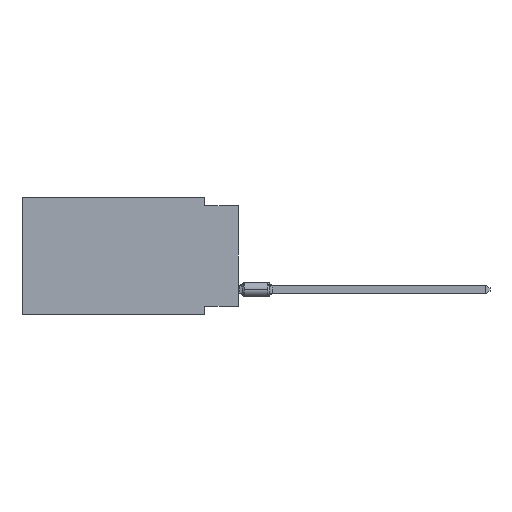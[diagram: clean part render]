
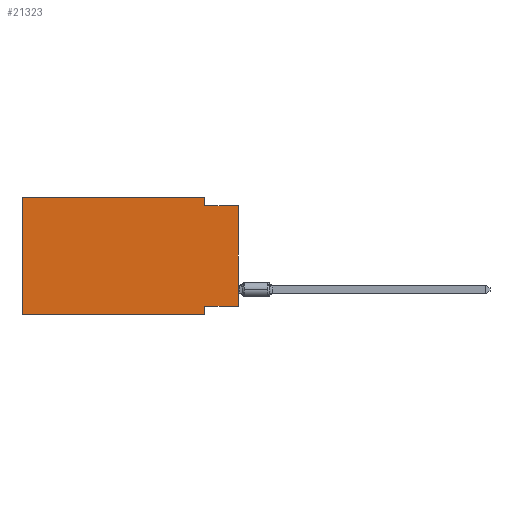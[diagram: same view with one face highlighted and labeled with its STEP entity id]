
A CAD part, left-side view. The second image highlights one B-rep face of the part: STEP entity #21323.
In plain terms, the highlighted planar face has unit normal (-1, 0, 0).
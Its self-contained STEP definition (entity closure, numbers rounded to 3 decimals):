
#197 = CARTESIAN_POINT ( 'NONE',  ( 0., 0., -0.635 ) ) ;
#879 = ORIENTED_EDGE ( 'NONE', *, *, #2220, .F. ) ;
#1951 = VECTOR ( 'NONE', #9381, 1000. ) ;
#2060 = CARTESIAN_POINT ( 'NONE',  ( 0., 2.54, -8.89 ) ) ;
#2220 = EDGE_CURVE ( 'NONE', #26242, #5443, #21758, .T. ) ;
#3222 = DIRECTION ( 'NONE',  ( 0., 0., -1. ) ) ;
#3522 = ORIENTED_EDGE ( 'NONE', *, *, #27773, .F. ) ;
#3531 = CARTESIAN_POINT ( 'NONE',  ( 0., 0., -8.255 ) ) ;
#5067 = CARTESIAN_POINT ( 'NONE',  ( 0., 16.383, 0. ) ) ;
#5443 = VERTEX_POINT ( 'NONE', #11147 ) ;
#5826 = LINE ( 'NONE', #3531, #21915 ) ;
#6061 = VERTEX_POINT ( 'NONE', #25067 ) ;
#6140 = CARTESIAN_POINT ( 'NONE',  ( 0., 0., 0. ) ) ;
#6212 = VERTEX_POINT ( 'NONE', #23338 ) ;
#6321 = VECTOR ( 'NONE', #11438, 1000. ) ;
#6931 = LINE ( 'NONE', #5067, #1951 ) ;
#7068 = CARTESIAN_POINT ( 'NONE',  ( 0., 0., -8.255 ) ) ;
#8894 = LINE ( 'NONE', #13213, #27435 ) ;
#9102 = DIRECTION ( 'NONE',  ( 0., 0., -1. ) ) ;
#9381 = DIRECTION ( 'NONE',  ( 0., 0., 1. ) ) ;
#9440 = ORIENTED_EDGE ( 'NONE', *, *, #27808, .F. ) ;
#9858 = DIRECTION ( 'NONE',  ( 0., 1., 0. ) ) ;
#10807 = VERTEX_POINT ( 'NONE', #12967 ) ;
#10947 = ORIENTED_EDGE ( 'NONE', *, *, #16075, .T. ) ;
#10988 = ORIENTED_EDGE ( 'NONE', *, *, #23152, .F. ) ;
#11147 = CARTESIAN_POINT ( 'NONE',  ( 0., 2.54, -8.89 ) ) ;
#11438 = DIRECTION ( 'NONE',  ( 0., -1., 0. ) ) ;
#12354 = VERTEX_POINT ( 'NONE', #7068 ) ;
#12698 = VECTOR ( 'NONE', #27195, 1000. ) ;
#12967 = CARTESIAN_POINT ( 'NONE',  ( 0., 16.383, 0. ) ) ;
#13213 = CARTESIAN_POINT ( 'NONE',  ( 0., 16.383, 0. ) ) ;
#13709 = EDGE_LOOP ( 'NONE', ( #16126, #23809, #3522, #10988, #9440, #10947, #879, #17304 ) ) ;
#14358 = VECTOR ( 'NONE', #27237, 1000. ) ;
#14563 = FACE_OUTER_BOUND ( 'NONE', #13709, .T. ) ;
#16075 = EDGE_CURVE ( 'NONE', #6212, #5443, #20333, .T. ) ;
#16126 = ORIENTED_EDGE ( 'NONE', *, *, #28358, .T. ) ;
#16283 = LINE ( 'NONE', #18000, #14358 ) ;
#17304 = ORIENTED_EDGE ( 'NONE', *, *, #20858, .F. ) ;
#17665 = DIRECTION ( 'NONE',  ( 0., -1., 0. ) ) ;
#17856 = VECTOR ( 'NONE', #9102, 1000. ) ;
#18000 = CARTESIAN_POINT ( 'NONE',  ( 0., 2.54, 0. ) ) ;
#18242 = AXIS2_PLACEMENT_3D ( 'NONE', #24934, #22922, #3222 ) ;
#18428 = EDGE_CURVE ( 'NONE', #20421, #21186, #18538, .T. ) ;
#18538 = LINE ( 'NONE', #20403, #12698 ) ;
#19218 = DIRECTION ( 'NONE',  ( 0., 0., 1. ) ) ;
#20333 = LINE ( 'NONE', #26401, #6321 ) ;
#20403 = CARTESIAN_POINT ( 'NONE',  ( 0., 0., -0.635 ) ) ;
#20421 = VERTEX_POINT ( 'NONE', #24693 ) ;
#20858 = EDGE_CURVE ( 'NONE', #12354, #26242, #5826, .T. ) ;
#20903 = PLANE ( 'NONE',  #18242 ) ;
#21113 = LINE ( 'NONE', #6140, #23110 ) ;
#21186 = VERTEX_POINT ( 'NONE', #197 ) ;
#21323 = ADVANCED_FACE ( 'NONE', ( #14563 ), #20903, .F. ) ;
#21758 = LINE ( 'NONE', #2060, #17856 ) ;
#21915 = VECTOR ( 'NONE', #9858, 1000. ) ;
#22922 = DIRECTION ( 'NONE',  ( 1., 0., 0. ) ) ;
#23110 = VECTOR ( 'NONE', #19218, 1000. ) ;
#23152 = EDGE_CURVE ( 'NONE', #10807, #6061, #8894, .T. ) ;
#23338 = CARTESIAN_POINT ( 'NONE',  ( 0., 16.383, -8.89 ) ) ;
#23809 = ORIENTED_EDGE ( 'NONE', *, *, #18428, .F. ) ;
#24166 = CARTESIAN_POINT ( 'NONE',  ( 0., 2.54, -8.255 ) ) ;
#24693 = CARTESIAN_POINT ( 'NONE',  ( 0., 2.54, -0.635 ) ) ;
#24934 = CARTESIAN_POINT ( 'NONE',  ( 0., 16.383, 0. ) ) ;
#25067 = CARTESIAN_POINT ( 'NONE',  ( 0., 2.54, 0. ) ) ;
#26242 = VERTEX_POINT ( 'NONE', #24166 ) ;
#26401 = CARTESIAN_POINT ( 'NONE',  ( 0., 16.383, -8.89 ) ) ;
#27195 = DIRECTION ( 'NONE',  ( 0., -1., 0. ) ) ;
#27237 = DIRECTION ( 'NONE',  ( 0., 0., -1. ) ) ;
#27435 = VECTOR ( 'NONE', #17665, 1000. ) ;
#27773 = EDGE_CURVE ( 'NONE', #6061, #20421, #16283, .T. ) ;
#27808 = EDGE_CURVE ( 'NONE', #6212, #10807, #6931, .T. ) ;
#28358 = EDGE_CURVE ( 'NONE', #12354, #21186, #21113, .T. ) ;
